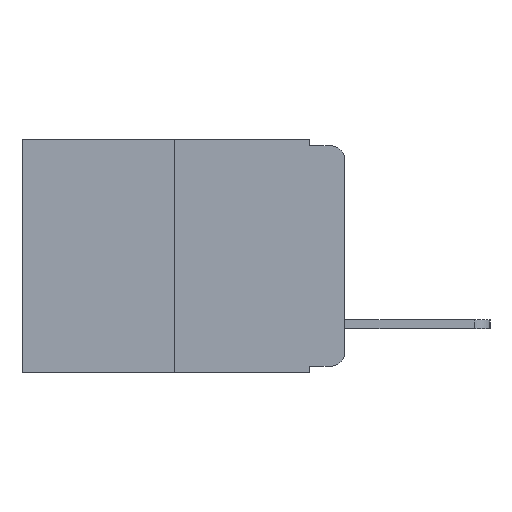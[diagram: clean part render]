
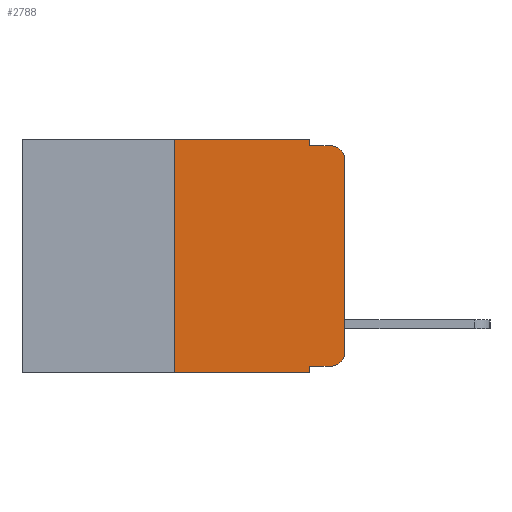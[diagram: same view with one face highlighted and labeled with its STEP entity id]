
A CAD part, left-side view. The second image highlights one B-rep face of the part: STEP entity #2788.
In plain terms, the highlighted planar face has unit normal (-1, 0, 0).
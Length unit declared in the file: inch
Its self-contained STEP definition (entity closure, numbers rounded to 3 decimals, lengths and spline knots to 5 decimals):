
#10 = VERTEX_POINT ( 'NONE', #5045 ) ;
#48 = VERTEX_POINT ( 'NONE', #10414 ) ;
#103 = ORIENTED_EDGE ( 'NONE', *, *, #11197, .F. ) ;
#229 = EDGE_CURVE ( 'NONE', #7282, #11387, #12506, .T. ) ;
#489 = DIRECTION ( 'NONE',  ( 0., -1., 0. ) ) ;
#570 = DIRECTION ( 'NONE',  ( 0., -1., 0. ) ) ;
#622 = EDGE_CURVE ( 'NONE', #48, #11387, #1635, .T. ) ;
#817 = DIRECTION ( 'NONE',  ( 0., 0., -1. ) ) ;
#869 = DIRECTION ( 'NONE',  ( -1., 0., 0. ) ) ;
#930 = EDGE_CURVE ( 'NONE', #10150, #5946, #4327, .T. ) ;
#983 = CARTESIAN_POINT ( 'NONE',  ( 0., 0., 0. ) ) ;
#1099 = DIRECTION ( 'NONE',  ( -1., 0., 0. ) ) ;
#1446 = VECTOR ( 'NONE', #3097, 39.37008 ) ;
#1635 = LINE ( 'NONE', #11546, #11806 ) ;
#1661 = EDGE_CURVE ( 'NONE', #48, #10, #2476, .T. ) ;
#2476 = LINE ( 'NONE', #10916, #5306 ) ;
#2552 = ORIENTED_EDGE ( 'NONE', *, *, #9839, .T. ) ;
#2788 = ADVANCED_FACE ( 'NONE', ( #10734 ), #7058, .F. ) ;
#3097 = DIRECTION ( 'NONE',  ( 0., 0., 1. ) ) ;
#3173 = LINE ( 'NONE', #5683, #10636 ) ;
#3279 = ORIENTED_EDGE ( 'NONE', *, *, #930, .T. ) ;
#3334 = CARTESIAN_POINT ( 'NONE',  ( 0., 0.02, -0.01 ) ) ;
#4077 = CARTESIAN_POINT ( 'NONE',  ( 0., 0.473, 0. ) ) ;
#4149 = VECTOR ( 'NONE', #817, 39.37008 ) ;
#4167 = ORIENTED_EDGE ( 'NONE', *, *, #622, .T. ) ;
#4327 = LINE ( 'NONE', #983, #1446 ) ;
#4386 = ORIENTED_EDGE ( 'NONE', *, *, #11917, .F. ) ;
#5045 = CARTESIAN_POINT ( 'NONE',  ( 0., 0.25, 0. ) ) ;
#5092 = CARTESIAN_POINT ( 'NONE',  ( 0., 0.051, -0.343 ) ) ;
#5140 = DIRECTION ( 'NONE',  ( 0., 0., -1. ) ) ;
#5170 = CIRCLE ( 'NONE', #6253, 0.02 ) ;
#5261 = VERTEX_POINT ( 'NONE', #12788 ) ;
#5263 = EDGE_CURVE ( 'NONE', #5946, #6971, #5170, .T. ) ;
#5306 = VECTOR ( 'NONE', #8464, 39.37008 ) ;
#5469 = ORIENTED_EDGE ( 'NONE', *, *, #1661, .F. ) ;
#5683 = CARTESIAN_POINT ( 'NONE',  ( 0., 0.473, 0. ) ) ;
#5719 = LINE ( 'NONE', #8445, #10107 ) ;
#5932 = EDGE_CURVE ( 'NONE', #5261, #6375, #9559, .T. ) ;
#5946 = VERTEX_POINT ( 'NONE', #10804 ) ;
#6253 = AXIS2_PLACEMENT_3D ( 'NONE', #7307, #1099, #8232 ) ;
#6375 = VERTEX_POINT ( 'NONE', #11342 ) ;
#6404 = ORIENTED_EDGE ( 'NONE', *, *, #5932, .F. ) ;
#6409 = VERTEX_POINT ( 'NONE', #9509 ) ;
#6483 = ORIENTED_EDGE ( 'NONE', *, *, #5263, .T. ) ;
#6627 = DIRECTION ( 'NONE',  ( 0., -1., 0. ) ) ;
#6971 = VERTEX_POINT ( 'NONE', #3334 ) ;
#7058 = PLANE ( 'NONE',  #10521 ) ;
#7103 = CARTESIAN_POINT ( 'NONE',  ( 0., 0.02, -0.313 ) ) ;
#7282 = VERTEX_POINT ( 'NONE', #9701 ) ;
#7307 = CARTESIAN_POINT ( 'NONE',  ( 0., 0.02, -0.03 ) ) ;
#8027 = DIRECTION ( 'NONE',  ( 0., 0., -1. ) ) ;
#8028 = LINE ( 'NONE', #12378, #10210 ) ;
#8232 = DIRECTION ( 'NONE',  ( 0., 0., -1. ) ) ;
#8445 = CARTESIAN_POINT ( 'NONE',  ( 0., 0.051, -0.333 ) ) ;
#8464 = DIRECTION ( 'NONE',  ( 0., 0., 1. ) ) ;
#8582 = EDGE_CURVE ( 'NONE', #7282, #6409, #5719, .T. ) ;
#8790 = CIRCLE ( 'NONE', #8854, 0.02 ) ;
#8854 = AXIS2_PLACEMENT_3D ( 'NONE', #7103, #869, #8027 ) ;
#8880 = CARTESIAN_POINT ( 'NONE',  ( 0., 0.051, 0. ) ) ;
#9310 = CARTESIAN_POINT ( 'NONE',  ( 0., 0., -0.313 ) ) ;
#9509 = CARTESIAN_POINT ( 'NONE',  ( 0., 0.02, -0.333 ) ) ;
#9559 = LINE ( 'NONE', #8880, #4149 ) ;
#9617 = CARTESIAN_POINT ( 'NONE',  ( 0., 0.051, 0. ) ) ;
#9701 = CARTESIAN_POINT ( 'NONE',  ( 0., 0.051, -0.333 ) ) ;
#9740 = ORIENTED_EDGE ( 'NONE', *, *, #229, .F. ) ;
#9839 = EDGE_CURVE ( 'NONE', #6409, #10150, #8790, .T. ) ;
#10045 = VECTOR ( 'NONE', #10332, 39.37008 ) ;
#10107 = VECTOR ( 'NONE', #6627, 39.37008 ) ;
#10150 = VERTEX_POINT ( 'NONE', #9310 ) ;
#10210 = VECTOR ( 'NONE', #570, 39.37008 ) ;
#10222 = ORIENTED_EDGE ( 'NONE', *, *, #8582, .T. ) ;
#10332 = DIRECTION ( 'NONE',  ( 0., 0., -1. ) ) ;
#10363 = DIRECTION ( 'NONE',  ( 0., -1., 0. ) ) ;
#10414 = CARTESIAN_POINT ( 'NONE',  ( 0., 0.25, -0.343 ) ) ;
#10505 = EDGE_LOOP ( 'NONE', ( #3279, #6483, #103, #6404, #4386, #5469, #4167, #9740, #10222, #2552 ) ) ;
#10521 = AXIS2_PLACEMENT_3D ( 'NONE', #4077, #10794, #5140 ) ;
#10636 = VECTOR ( 'NONE', #10363, 39.37008 ) ;
#10734 = FACE_OUTER_BOUND ( 'NONE', #10505, .T. ) ;
#10794 = DIRECTION ( 'NONE',  ( 1., 0., 0. ) ) ;
#10804 = CARTESIAN_POINT ( 'NONE',  ( 0., 0., -0.03 ) ) ;
#10916 = CARTESIAN_POINT ( 'NONE',  ( 0., 0.25, 0. ) ) ;
#11197 = EDGE_CURVE ( 'NONE', #6375, #6971, #8028, .T. ) ;
#11342 = CARTESIAN_POINT ( 'NONE',  ( 0., 0.051, -0.01 ) ) ;
#11387 = VERTEX_POINT ( 'NONE', #5092 ) ;
#11546 = CARTESIAN_POINT ( 'NONE',  ( 0., 0.473, -0.343 ) ) ;
#11806 = VECTOR ( 'NONE', #489, 39.37008 ) ;
#11917 = EDGE_CURVE ( 'NONE', #10, #5261, #3173, .T. ) ;
#12378 = CARTESIAN_POINT ( 'NONE',  ( 0., 0.051, -0.01 ) ) ;
#12506 = LINE ( 'NONE', #9617, #10045 ) ;
#12788 = CARTESIAN_POINT ( 'NONE',  ( 0., 0.051, 0. ) ) ;
